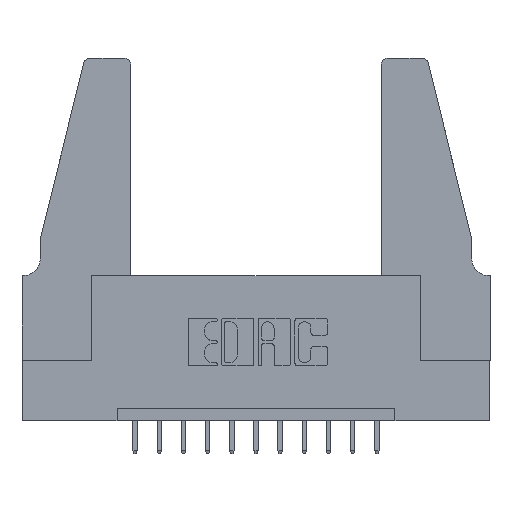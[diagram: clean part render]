
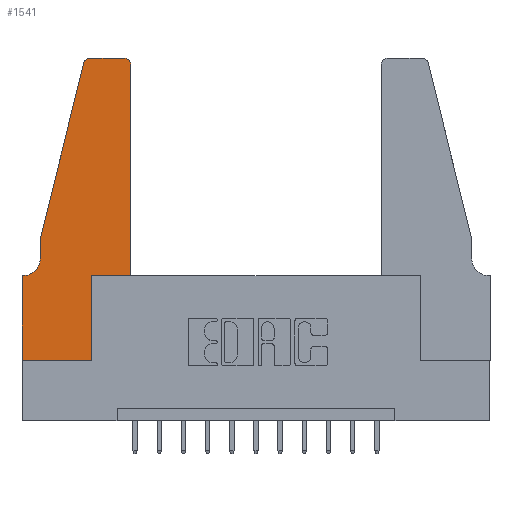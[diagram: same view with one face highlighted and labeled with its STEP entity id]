
A CAD part, top view. The second image highlights one B-rep face of the part: STEP entity #1541.
In plain terms, the highlighted planar face has unit normal (0, 0, 1).
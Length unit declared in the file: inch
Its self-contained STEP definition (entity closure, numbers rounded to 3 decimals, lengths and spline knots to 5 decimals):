
#28 = CARTESIAN_POINT ( 'NONE',  ( 0.2865, 0., 0.37 ) ) ;
#47 = EDGE_CURVE ( 'NONE', #8313, #11711, #790, .T. ) ;
#62 = DIRECTION ( 'NONE',  ( 1., 0., 0. ) ) ;
#156 = CARTESIAN_POINT ( 'NONE',  ( 0., 0., 0.37 ) ) ;
#549 = CARTESIAN_POINT ( 'NONE',  ( 0.4505, 0.35, 0.37 ) ) ;
#589 = CARTESIAN_POINT ( 'NONE',  ( 0.284, 1.22, 0.37 ) ) ;
#634 = DIRECTION ( 'NONE',  ( -1., 0., 0. ) ) ;
#699 = CARTESIAN_POINT ( 'NONE',  ( 0.2605, 1.25, 0.37 ) ) ;
#772 = LINE ( 'NONE', #699, #7392 ) ;
#790 = LINE ( 'NONE', #2820, #8775 ) ;
#925 = CARTESIAN_POINT ( 'NONE',  ( 0.0755, 0.35, 0.37 ) ) ;
#1277 = CARTESIAN_POINT ( 'NONE',  ( 0.0055, 0.35, 0.37 ) ) ;
#1487 = EDGE_CURVE ( 'NONE', #4967, #3869, #10220, .T. ) ;
#1541 = ADVANCED_FACE ( 'NONE', ( #7184 ), #10559, .T. ) ;
#2066 = ORIENTED_EDGE ( 'NONE', *, *, #3957, .T. ) ;
#2183 = LINE ( 'NONE', #3531, #4772 ) ;
#2275 = CARTESIAN_POINT ( 'NONE',  ( 0.4205, 1.22, 0.37 ) ) ;
#2359 = DIRECTION ( 'NONE',  ( 1., 0., 0. ) ) ;
#2468 = VERTEX_POINT ( 'NONE', #1277 ) ;
#2522 = ORIENTED_EDGE ( 'NONE', *, *, #8485, .T. ) ;
#2605 = AXIS2_PLACEMENT_3D ( 'NONE', #13078, #2846, #634 ) ;
#2664 = CIRCLE ( 'NONE', #5271, 0.03 ) ;
#2768 = EDGE_CURVE ( 'NONE', #2468, #9663, #6450, .T. ) ;
#2820 = CARTESIAN_POINT ( 'NONE',  ( 0.0755, 0.5, 0.37 ) ) ;
#2846 = DIRECTION ( 'NONE',  ( 0., 0., -1. ) ) ;
#2945 = EDGE_CURVE ( 'NONE', #9916, #3910, #2664, .T. ) ;
#3182 = EDGE_LOOP ( 'NONE', ( #12983, #4453, #9952, #2066, #5808, #7434, #7968, #10806, #2522, #13418, #3924, #4890 ) ) ;
#3396 = VECTOR ( 'NONE', #10299, 39.37008 ) ;
#3453 = CARTESIAN_POINT ( 'NONE',  ( 0.0755, 0.5, 0.37 ) ) ;
#3531 = CARTESIAN_POINT ( 'NONE',  ( 0., 0., 0.37 ) ) ;
#3869 = VERTEX_POINT ( 'NONE', #28 ) ;
#3910 = VERTEX_POINT ( 'NONE', #4500 ) ;
#3924 = ORIENTED_EDGE ( 'NONE', *, *, #12928, .T. ) ;
#3957 = EDGE_CURVE ( 'NONE', #11711, #4079, #6937, .T. ) ;
#4045 = CARTESIAN_POINT ( 'NONE',  ( 0.25487, 1.22718, 0.37 ) ) ;
#4054 = LINE ( 'NONE', #549, #13686 ) ;
#4079 = VERTEX_POINT ( 'NONE', #7048 ) ;
#4104 = EDGE_CURVE ( 'NONE', #8400, #7024, #13815, .T. ) ;
#4228 = DIRECTION ( 'NONE',  ( -0.239, -0.971, 0. ) ) ;
#4453 = ORIENTED_EDGE ( 'NONE', *, *, #9995, .T. ) ;
#4500 = CARTESIAN_POINT ( 'NONE',  ( 0.4205, 1.25, 0.37 ) ) ;
#4772 = VECTOR ( 'NONE', #8045, 39.37008 ) ;
#4890 = ORIENTED_EDGE ( 'NONE', *, *, #2945, .T. ) ;
#4967 = VERTEX_POINT ( 'NONE', #156 ) ;
#5271 = AXIS2_PLACEMENT_3D ( 'NONE', #2275, #5859, #2359 ) ;
#5808 = ORIENTED_EDGE ( 'NONE', *, *, #6596, .T. ) ;
#5859 = DIRECTION ( 'NONE',  ( 0., 0., 1. ) ) ;
#5934 = CIRCLE ( 'NONE', #2605, 0.07 ) ;
#6450 = LINE ( 'NONE', #925, #9026 ) ;
#6463 = DIRECTION ( 'NONE',  ( 1., 0., 0. ) ) ;
#6480 = CIRCLE ( 'NONE', #10720, 0.03 ) ;
#6596 = EDGE_CURVE ( 'NONE', #4079, #2468, #5934, .T. ) ;
#6937 = LINE ( 'NONE', #3453, #7658 ) ;
#7024 = VERTEX_POINT ( 'NONE', #12831 ) ;
#7048 = CARTESIAN_POINT ( 'NONE',  ( 0.0755, 0.42, 0.37 ) ) ;
#7184 = FACE_OUTER_BOUND ( 'NONE', #3182, .T. ) ;
#7392 = VECTOR ( 'NONE', #9953, 39.37008 ) ;
#7434 = ORIENTED_EDGE ( 'NONE', *, *, #2768, .T. ) ;
#7658 = VECTOR ( 'NONE', #13531, 39.37008 ) ;
#7874 = AXIS2_PLACEMENT_3D ( 'NONE', #9538, #14009, #9605 ) ;
#7937 = EDGE_CURVE ( 'NONE', #3910, #14489, #772, .T. ) ;
#7968 = ORIENTED_EDGE ( 'NONE', *, *, #8109, .T. ) ;
#8045 = DIRECTION ( 'NONE',  ( 0., -1., 0. ) ) ;
#8109 = EDGE_CURVE ( 'NONE', #9663, #4967, #2183, .T. ) ;
#8247 = CARTESIAN_POINT ( 'NONE',  ( 0.284, 1.25, 0.37 ) ) ;
#8313 = VERTEX_POINT ( 'NONE', #4045 ) ;
#8400 = VERTEX_POINT ( 'NONE', #11272 ) ;
#8485 = EDGE_CURVE ( 'NONE', #3869, #8400, #11350, .T. ) ;
#8775 = VECTOR ( 'NONE', #4228, 39.37008 ) ;
#9026 = VECTOR ( 'NONE', #13129, 39.37008 ) ;
#9049 = CARTESIAN_POINT ( 'NONE',  ( 0.2865, 0.35, 0.37 ) ) ;
#9120 = DIRECTION ( 'NONE',  ( 0., 1., 0. ) ) ;
#9538 = CARTESIAN_POINT ( 'NONE',  ( 0., 0.35, 0.37 ) ) ;
#9605 = DIRECTION ( 'NONE',  ( 1., 0., 0. ) ) ;
#9629 = DIRECTION ( 'NONE',  ( 0., 0., 1. ) ) ;
#9663 = VERTEX_POINT ( 'NONE', #12634 ) ;
#9916 = VERTEX_POINT ( 'NONE', #10959 ) ;
#9952 = ORIENTED_EDGE ( 'NONE', *, *, #47, .T. ) ;
#9953 = DIRECTION ( 'NONE',  ( -1., 0., 0. ) ) ;
#9995 = EDGE_CURVE ( 'NONE', #14489, #8313, #6480, .T. ) ;
#10220 = LINE ( 'NONE', #14561, #12145 ) ;
#10299 = DIRECTION ( 'NONE',  ( 1., 0., 0. ) ) ;
#10559 = PLANE ( 'NONE',  #7874 ) ;
#10720 = AXIS2_PLACEMENT_3D ( 'NONE', #589, #9629, #6463 ) ;
#10806 = ORIENTED_EDGE ( 'NONE', *, *, #1487, .T. ) ;
#10959 = CARTESIAN_POINT ( 'NONE',  ( 0.4505, 1.22, 0.37 ) ) ;
#11272 = CARTESIAN_POINT ( 'NONE',  ( 0.2865, 0.35, 0.37 ) ) ;
#11350 = LINE ( 'NONE', #9049, #11898 ) ;
#11353 = CARTESIAN_POINT ( 'NONE',  ( 0.0755, 0.5, 0.37 ) ) ;
#11711 = VERTEX_POINT ( 'NONE', #11353 ) ;
#11898 = VECTOR ( 'NONE', #9120, 39.37008 ) ;
#12145 = VECTOR ( 'NONE', #62, 39.37008 ) ;
#12634 = CARTESIAN_POINT ( 'NONE',  ( 0., 0.35, 0.37 ) ) ;
#12690 = CARTESIAN_POINT ( 'NONE',  ( 0.4505, 0.35, 0.37 ) ) ;
#12831 = CARTESIAN_POINT ( 'NONE',  ( 0.4505, 0.35, 0.37 ) ) ;
#12928 = EDGE_CURVE ( 'NONE', #7024, #9916, #4054, .T. ) ;
#12983 = ORIENTED_EDGE ( 'NONE', *, *, #7937, .T. ) ;
#13078 = CARTESIAN_POINT ( 'NONE',  ( 0.0055, 0.42, 0.37 ) ) ;
#13129 = DIRECTION ( 'NONE',  ( -1., 0., 0. ) ) ;
#13418 = ORIENTED_EDGE ( 'NONE', *, *, #4104, .T. ) ;
#13531 = DIRECTION ( 'NONE',  ( 0., -1., 0. ) ) ;
#13686 = VECTOR ( 'NONE', #14298, 39.37008 ) ;
#13815 = LINE ( 'NONE', #12690, #3396 ) ;
#14009 = DIRECTION ( 'NONE',  ( 0., 0., 1. ) ) ;
#14298 = DIRECTION ( 'NONE',  ( 0., 1., 0. ) ) ;
#14489 = VERTEX_POINT ( 'NONE', #8247 ) ;
#14561 = CARTESIAN_POINT ( 'NONE',  ( 0., 0., 0.37 ) ) ;
